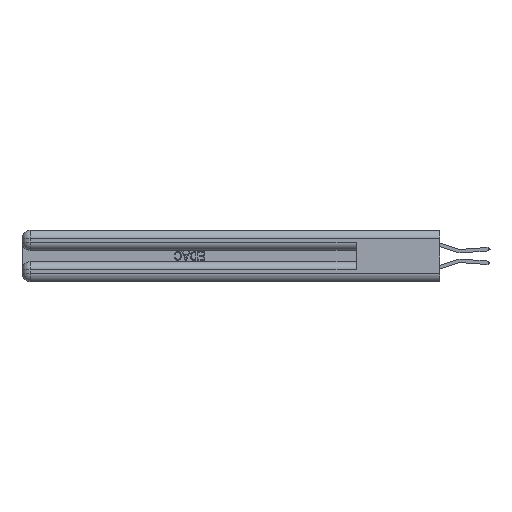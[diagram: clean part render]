
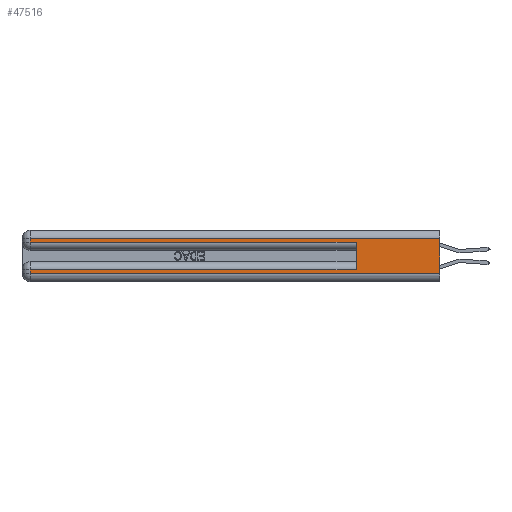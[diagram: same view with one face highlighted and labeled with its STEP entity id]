
A CAD part, left-side view. The second image highlights one B-rep face of the part: STEP entity #47516.
In plain terms, the highlighted planar face has unit normal (-1, 0, 0).
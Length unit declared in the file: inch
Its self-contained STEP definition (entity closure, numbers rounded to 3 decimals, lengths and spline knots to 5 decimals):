
#1306 = VERTEX_POINT ( 'NONE', #18996 ) ;
#1758 = VERTEX_POINT ( 'NONE', #25571 ) ;
#2216 = VERTEX_POINT ( 'NONE', #39311 ) ;
#3309 = DIRECTION ( 'NONE',  ( 0., 1., 0. ) ) ;
#3628 = DIRECTION ( 'NONE',  ( 0., 0., -1. ) ) ;
#3629 = ORIENTED_EDGE ( 'NONE', *, *, #27916, .T. ) ;
#3737 = DIRECTION ( 'NONE',  ( 0., 0., 1. ) ) ;
#4472 = EDGE_LOOP ( 'NONE', ( #7879, #20597, #21794, #11399, #42762, #6024, #7863, #3629 ) ) ;
#5117 = CARTESIAN_POINT ( 'NONE',  ( 0., 0., 0.06 ) ) ;
#5396 = DIRECTION ( 'NONE',  ( 0., 1., 0. ) ) ;
#5593 = CARTESIAN_POINT ( 'NONE',  ( 0., 2.94, 0.285 ) ) ;
#6024 = ORIENTED_EDGE ( 'NONE', *, *, #48144, .T. ) ;
#6847 = DIRECTION ( 'NONE',  ( 0., 0., -1. ) ) ;
#7583 = CARTESIAN_POINT ( 'NONE',  ( 0., 0., 0.37 ) ) ;
#7863 = ORIENTED_EDGE ( 'NONE', *, *, #34309, .T. ) ;
#7879 = ORIENTED_EDGE ( 'NONE', *, *, #27168, .F. ) ;
#11098 = CARTESIAN_POINT ( 'NONE',  ( 0., 0., 0.085 ) ) ;
#11399 = ORIENTED_EDGE ( 'NONE', *, *, #33947, .T. ) ;
#11683 = LINE ( 'NONE', #40082, #41207 ) ;
#12350 = VECTOR ( 'NONE', #6847, 39.37008 ) ;
#13844 = VERTEX_POINT ( 'NONE', #20010 ) ;
#14481 = CARTESIAN_POINT ( 'NONE',  ( 0., 2.94, 0.37 ) ) ;
#15372 = CARTESIAN_POINT ( 'NONE',  ( 0., 0., 0.37 ) ) ;
#15429 = CARTESIAN_POINT ( 'NONE',  ( 0., 0.6, 0.145 ) ) ;
#15862 = EDGE_CURVE ( 'NONE', #13844, #49392, #35304, .T. ) ;
#16496 = VECTOR ( 'NONE', #3628, 39.37008 ) ;
#16687 = VECTOR ( 'NONE', #5396, 39.37008 ) ;
#18996 = CARTESIAN_POINT ( 'NONE',  ( 0., 0.6, 0.085 ) ) ;
#19275 = DIRECTION ( 'NONE',  ( 1., 0., 0. ) ) ;
#19734 = FACE_OUTER_BOUND ( 'NONE', #4472, .T. ) ;
#20010 = CARTESIAN_POINT ( 'NONE',  ( 0., 2.94, 0.31 ) ) ;
#20597 = ORIENTED_EDGE ( 'NONE', *, *, #47797, .T. ) ;
#20764 = CARTESIAN_POINT ( 'NONE',  ( 0., 2.94, 0.085 ) ) ;
#21794 = ORIENTED_EDGE ( 'NONE', *, *, #15862, .T. ) ;
#24656 = CARTESIAN_POINT ( 'NONE',  ( 0., 0., 0.31 ) ) ;
#24746 = LINE ( 'NONE', #15429, #43979 ) ;
#25571 = CARTESIAN_POINT ( 'NONE',  ( 0., 0., 0.31 ) ) ;
#25573 = LINE ( 'NONE', #26793, #16496 ) ;
#26793 = CARTESIAN_POINT ( 'NONE',  ( 0., 2.94, 0.37 ) ) ;
#26958 = LINE ( 'NONE', #24656, #16687 ) ;
#27168 = EDGE_CURVE ( 'NONE', #1758, #41663, #40403, .T. ) ;
#27547 = EDGE_CURVE ( 'NONE', #1306, #39909, #24746, .T. ) ;
#27916 = EDGE_CURVE ( 'NONE', #2216, #41663, #37349, .T. ) ;
#28999 = VECTOR ( 'NONE', #38472, 39.37008 ) ;
#32528 = DIRECTION ( 'NONE',  ( 0., -1., 0. ) ) ;
#33947 = EDGE_CURVE ( 'NONE', #49392, #39909, #11683, .T. ) ;
#34309 = EDGE_CURVE ( 'NONE', #47787, #2216, #25573, .T. ) ;
#35304 = LINE ( 'NONE', #14481, #12350 ) ;
#35804 = AXIS2_PLACEMENT_3D ( 'NONE', #7583, #19275, #46185 ) ;
#36152 = VECTOR ( 'NONE', #49411, 39.37008 ) ;
#37349 = LINE ( 'NONE', #45509, #36152 ) ;
#38472 = DIRECTION ( 'NONE',  ( 0., 0., -1. ) ) ;
#39311 = CARTESIAN_POINT ( 'NONE',  ( 0., 2.94, 0.06 ) ) ;
#39909 = VERTEX_POINT ( 'NONE', #47879 ) ;
#40082 = CARTESIAN_POINT ( 'NONE',  ( 0., 0., 0.285 ) ) ;
#40403 = LINE ( 'NONE', #15372, #28999 ) ;
#41207 = VECTOR ( 'NONE', #32528, 39.37008 ) ;
#41663 = VERTEX_POINT ( 'NONE', #5117 ) ;
#41921 = VECTOR ( 'NONE', #3309, 39.37008 ) ;
#42307 = PLANE ( 'NONE',  #35804 ) ;
#42762 = ORIENTED_EDGE ( 'NONE', *, *, #27547, .F. ) ;
#43153 = LINE ( 'NONE', #11098, #41921 ) ;
#43979 = VECTOR ( 'NONE', #3737, 39.37008 ) ;
#45509 = CARTESIAN_POINT ( 'NONE',  ( 0., 0., 0.06 ) ) ;
#46185 = DIRECTION ( 'NONE',  ( 0., 0., -1. ) ) ;
#47516 = ADVANCED_FACE ( 'NONE', ( #19734 ), #42307, .F. ) ;
#47787 = VERTEX_POINT ( 'NONE', #20764 ) ;
#47797 = EDGE_CURVE ( 'NONE', #1758, #13844, #26958, .T. ) ;
#47879 = CARTESIAN_POINT ( 'NONE',  ( 0., 0.6, 0.285 ) ) ;
#48144 = EDGE_CURVE ( 'NONE', #1306, #47787, #43153, .T. ) ;
#49392 = VERTEX_POINT ( 'NONE', #5593 ) ;
#49411 = DIRECTION ( 'NONE',  ( 0., -1., 0. ) ) ;
